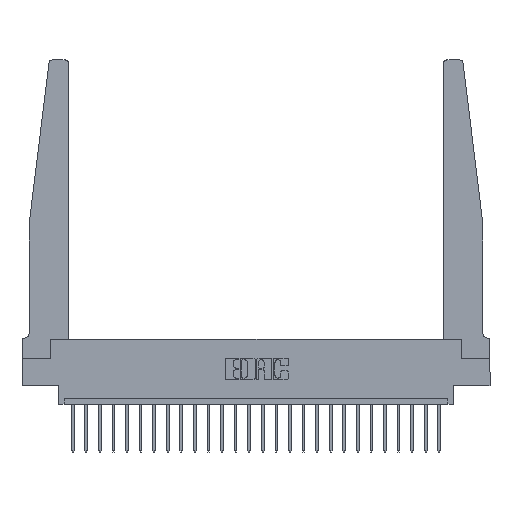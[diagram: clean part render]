
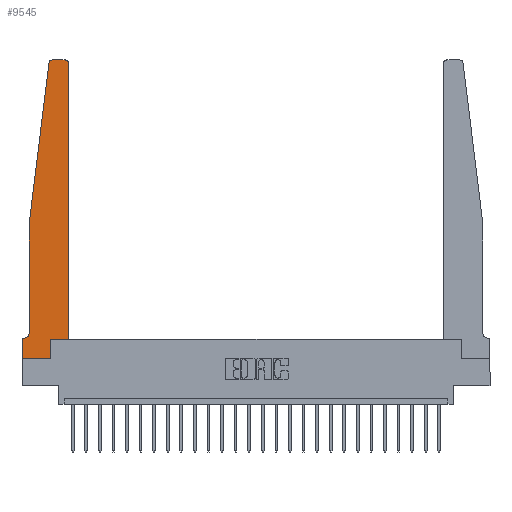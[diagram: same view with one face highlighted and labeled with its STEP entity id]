
A CAD part, top view. The second image highlights one B-rep face of the part: STEP entity #9545.
In plain terms, the highlighted planar face has unit normal (0, 0, 1).
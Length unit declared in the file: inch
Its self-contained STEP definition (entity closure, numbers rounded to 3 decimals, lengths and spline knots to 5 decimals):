
#363 = DIRECTION ( 'NONE',  ( 1., 0., 0. ) ) ;
#444 = VERTEX_POINT ( 'NONE', #8802 ) ;
#468 = ORIENTED_EDGE ( 'NONE', *, *, #18547, .T. ) ;
#647 = CARTESIAN_POINT ( 'NONE',  ( 0.2605, 0.18, 0.37 ) ) ;
#684 = CARTESIAN_POINT ( 'NONE',  ( 0.395, 2.75, 0.37 ) ) ;
#1386 = VERTEX_POINT ( 'NONE', #22783 ) ;
#1800 = EDGE_CURVE ( 'NONE', #1386, #23972, #23453, .T. ) ;
#1802 = EDGE_CURVE ( 'NONE', #23972, #19198, #16753, .T. ) ;
#1853 = CARTESIAN_POINT ( 'NONE',  ( 0., 0.1875, 0.37 ) ) ;
#2974 = VECTOR ( 'NONE', #24038, 39.37008 ) ;
#2986 = AXIS2_PLACEMENT_3D ( 'NONE', #23868, #20178, #22125 ) ;
#3236 = DIRECTION ( 'NONE',  ( -0.122, -0.992, 0. ) ) ;
#3560 = ORIENTED_EDGE ( 'NONE', *, *, #5492, .T. ) ;
#3577 = PLANE ( 'NONE',  #2986 ) ;
#4020 = LINE ( 'NONE', #15389, #11530 ) ;
#5032 = ORIENTED_EDGE ( 'NONE', *, *, #17712, .T. ) ;
#5036 = DIRECTION ( 'NONE',  ( -1., 0., 0. ) ) ;
#5056 = ORIENTED_EDGE ( 'NONE', *, *, #10725, .T. ) ;
#5492 = EDGE_CURVE ( 'NONE', #15237, #5771, #12905, .T. ) ;
#5610 = VERTEX_POINT ( 'NONE', #13606 ) ;
#5677 = DIRECTION ( 'NONE',  ( 1., 0., 0. ) ) ;
#5771 = VERTEX_POINT ( 'NONE', #16369 ) ;
#5990 = EDGE_CURVE ( 'NONE', #5771, #444, #4020, .T. ) ;
#6001 = ORIENTED_EDGE ( 'NONE', *, *, #20267, .T. ) ;
#6728 = VECTOR ( 'NONE', #6804, 39.37008 ) ;
#6785 = CARTESIAN_POINT ( 'NONE',  ( 0.425, 0.18, 0.37 ) ) ;
#6804 = DIRECTION ( 'NONE',  ( -1., 0., 0. ) ) ;
#6825 = VECTOR ( 'NONE', #5677, 39.37008 ) ;
#6840 = CARTESIAN_POINT ( 'NONE',  ( 0.015, 0.2375, 0.37 ) ) ;
#7034 = LINE ( 'NONE', #6785, #10767 ) ;
#7177 = ORIENTED_EDGE ( 'NONE', *, *, #12021, .T. ) ;
#7352 = CIRCLE ( 'NONE', #20895, 0.03 ) ;
#7411 = VECTOR ( 'NONE', #3236, 39.37008 ) ;
#7606 = VERTEX_POINT ( 'NONE', #10055 ) ;
#7651 = FACE_OUTER_BOUND ( 'NONE', #11409, .T. ) ;
#8209 = LINE ( 'NONE', #18814, #16938 ) ;
#8419 = EDGE_CURVE ( 'NONE', #444, #1386, #12615, .T. ) ;
#8632 = CIRCLE ( 'NONE', #12344, 0.03 ) ;
#8701 = DIRECTION ( 'NONE',  ( 0., 0., -1. ) ) ;
#8802 = CARTESIAN_POINT ( 'NONE',  ( 0.065, 0.2375, 0.37 ) ) ;
#9481 = AXIS2_PLACEMENT_3D ( 'NONE', #6840, #8701, #5036 ) ;
#9545 = ADVANCED_FACE ( 'NONE', ( #7651 ), #3577, .T. ) ;
#9683 = VERTEX_POINT ( 'NONE', #15386 ) ;
#9835 = DIRECTION ( 'NONE',  ( 0., -1., 0. ) ) ;
#9852 = VERTEX_POINT ( 'NONE', #684 ) ;
#9933 = DIRECTION ( 'NONE',  ( 0., 1., 0. ) ) ;
#10055 = CARTESIAN_POINT ( 'NONE',  ( 0.27653, 2.75, 0.37 ) ) ;
#10630 = CARTESIAN_POINT ( 'NONE',  ( 0.065, 1.25, 0.37 ) ) ;
#10725 = EDGE_CURVE ( 'NONE', #5610, #12338, #8209, .T. ) ;
#10767 = VECTOR ( 'NONE', #12275, 39.37008 ) ;
#10983 = CARTESIAN_POINT ( 'NONE',  ( 0.2605, 0.18, 0.37 ) ) ;
#11033 = LINE ( 'NONE', #17946, #6728 ) ;
#11409 = EDGE_LOOP ( 'NONE', ( #18784, #468, #3560, #13513, #21624, #16118, #23590, #5032, #6001, #7177, #5056, #21750 ) ) ;
#11528 = CARTESIAN_POINT ( 'NONE',  ( 0.27653, 2.72, 0.37 ) ) ;
#11530 = VECTOR ( 'NONE', #9835, 39.37008 ) ;
#11764 = VECTOR ( 'NONE', #20764, 39.37008 ) ;
#12021 = EDGE_CURVE ( 'NONE', #14688, #5610, #7034, .T. ) ;
#12178 = CARTESIAN_POINT ( 'NONE',  ( 0.065, 0.1875, 0.37 ) ) ;
#12275 = DIRECTION ( 'NONE',  ( 1., 0., 0. ) ) ;
#12338 = VERTEX_POINT ( 'NONE', #14795 ) ;
#12344 = AXIS2_PLACEMENT_3D ( 'NONE', #21808, #23715, #12518 ) ;
#12518 = DIRECTION ( 'NONE',  ( 1., 0., 0. ) ) ;
#12615 = CIRCLE ( 'NONE', #9481, 0.05 ) ;
#12905 = LINE ( 'NONE', #10630, #7411 ) ;
#13245 = DIRECTION ( 'NONE',  ( 0., 0., 1. ) ) ;
#13513 = ORIENTED_EDGE ( 'NONE', *, *, #5990, .T. ) ;
#13606 = CARTESIAN_POINT ( 'NONE',  ( 0.425, 0.18, 0.37 ) ) ;
#14035 = DIRECTION ( 'NONE',  ( -1., 0., 0. ) ) ;
#14688 = VERTEX_POINT ( 'NONE', #647 ) ;
#14795 = CARTESIAN_POINT ( 'NONE',  ( 0.425, 2.72, 0.37 ) ) ;
#15237 = VERTEX_POINT ( 'NONE', #23212 ) ;
#15386 = CARTESIAN_POINT ( 'NONE',  ( 0.2605, 0., 0.37 ) ) ;
#15389 = CARTESIAN_POINT ( 'NONE',  ( 0.065, 1.25, 0.37 ) ) ;
#16118 = ORIENTED_EDGE ( 'NONE', *, *, #1800, .T. ) ;
#16369 = CARTESIAN_POINT ( 'NONE',  ( 0.065, 1.25, 0.37 ) ) ;
#16753 = LINE ( 'NONE', #24121, #11764 ) ;
#16938 = VECTOR ( 'NONE', #9933, 39.37008 ) ;
#16950 = LINE ( 'NONE', #10983, #2974 ) ;
#17712 = EDGE_CURVE ( 'NONE', #19198, #9683, #23108, .T. ) ;
#17946 = CARTESIAN_POINT ( 'NONE',  ( 0.25, 2.75, 0.37 ) ) ;
#18470 = VECTOR ( 'NONE', #14035, 39.37008 ) ;
#18547 = EDGE_CURVE ( 'NONE', #7606, #15237, #7352, .T. ) ;
#18784 = ORIENTED_EDGE ( 'NONE', *, *, #20694, .T. ) ;
#18814 = CARTESIAN_POINT ( 'NONE',  ( 0.425, 0.18, 0.37 ) ) ;
#19198 = VERTEX_POINT ( 'NONE', #21016 ) ;
#20178 = DIRECTION ( 'NONE',  ( 0., 0., 1. ) ) ;
#20267 = EDGE_CURVE ( 'NONE', #9683, #14688, #16950, .T. ) ;
#20694 = EDGE_CURVE ( 'NONE', #9852, #7606, #11033, .T. ) ;
#20704 = CARTESIAN_POINT ( 'NONE',  ( 0., 0., 0.37 ) ) ;
#20764 = DIRECTION ( 'NONE',  ( 0., -1., 0. ) ) ;
#20895 = AXIS2_PLACEMENT_3D ( 'NONE', #11528, #13245, #363 ) ;
#21016 = CARTESIAN_POINT ( 'NONE',  ( 0., 0., 0.37 ) ) ;
#21624 = ORIENTED_EDGE ( 'NONE', *, *, #8419, .T. ) ;
#21750 = ORIENTED_EDGE ( 'NONE', *, *, #23395, .T. ) ;
#21808 = CARTESIAN_POINT ( 'NONE',  ( 0.395, 2.72, 0.37 ) ) ;
#22125 = DIRECTION ( 'NONE',  ( 1., 0., 0. ) ) ;
#22783 = CARTESIAN_POINT ( 'NONE',  ( 0.015, 0.1875, 0.37 ) ) ;
#23108 = LINE ( 'NONE', #20704, #6825 ) ;
#23212 = CARTESIAN_POINT ( 'NONE',  ( 0.24675, 2.72367, 0.37 ) ) ;
#23395 = EDGE_CURVE ( 'NONE', #12338, #9852, #8632, .T. ) ;
#23453 = LINE ( 'NONE', #12178, #18470 ) ;
#23590 = ORIENTED_EDGE ( 'NONE', *, *, #1802, .T. ) ;
#23715 = DIRECTION ( 'NONE',  ( 0., 0., 1. ) ) ;
#23868 = CARTESIAN_POINT ( 'NONE',  ( 0., 0.1875, 0.37 ) ) ;
#23972 = VERTEX_POINT ( 'NONE', #1853 ) ;
#24038 = DIRECTION ( 'NONE',  ( 0., 1., 0. ) ) ;
#24121 = CARTESIAN_POINT ( 'NONE',  ( 0., 0., 0.37 ) ) ;
